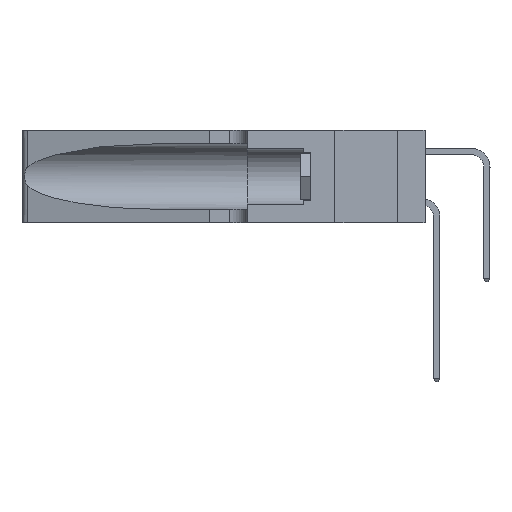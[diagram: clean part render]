
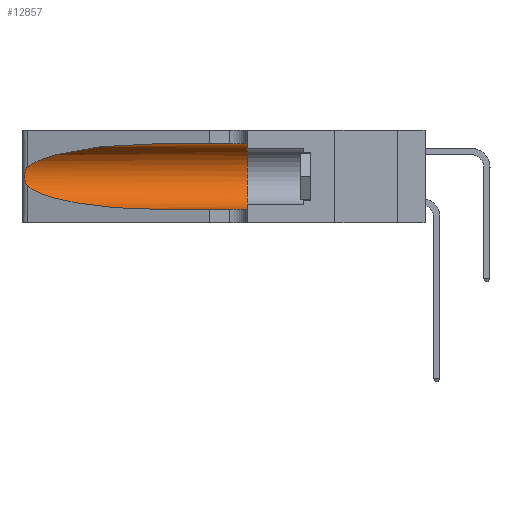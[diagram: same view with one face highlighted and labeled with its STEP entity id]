
A CAD part, left-side view. The second image highlights one B-rep face of the part: STEP entity #12857.
In plain terms, the highlighted cylindrical face has radius 3.308 mm (diameter 6.617 mm), a partial arc.
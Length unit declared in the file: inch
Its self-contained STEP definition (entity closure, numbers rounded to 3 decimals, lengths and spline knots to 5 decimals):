
#152 = CARTESIAN_POINT ( 'NONE',  ( 0.1305, 0.72297, 0.31525 ) ) ;
#205 = DIRECTION ( 'NONE',  ( 0., -1., 0. ) ) ;
#303 =( BOUNDED_CURVE ( )  B_SPLINE_CURVE ( 3, ( #8955, #23123, #22977, #10603 ),
 .UNSPECIFIED., .F., .F. ) 
 B_SPLINE_CURVE_WITH_KNOTS ( ( 4, 4 ),
 ( 3.44316, 4.71239 ),
 .UNSPECIFIED. ) 
 CURVE ( )  GEOMETRIC_REPRESENTATION_ITEM ( )  RATIONAL_B_SPLINE_CURVE ( ( 1., 0.87, 0.87, 1. ) ) 
 REPRESENTATION_ITEM ( '' )  );
#455 = ORIENTED_EDGE ( 'NONE', *, *, #1538, .T. ) ;
#816 = VERTEX_POINT ( 'NONE', #21031 ) ;
#879 = VERTEX_POINT ( 'NONE', #2943 ) ;
#1538 = EDGE_CURVE ( 'NONE', #21488, #879, #303, .T. ) ;
#2738 = CARTESIAN_POINT ( 'NONE',  ( 0.25787, 1.23484, 0.2124 ) ) ;
#2943 = CARTESIAN_POINT ( 'NONE',  ( 0.1305, 0.72297, 0.05475 ) ) ;
#3172 = LINE ( 'NONE', #18869, #17789 ) ;
#3259 = CARTESIAN_POINT ( 'NONE',  ( 0.1305, 0.35, 0.185 ) ) ;
#3769 = ORIENTED_EDGE ( 'NONE', *, *, #12923, .F. ) ;
#3780 = CARTESIAN_POINT ( 'NONE',  ( 0.1305, 1.61858, 0.185 ) ) ;
#3948 = EDGE_CURVE ( 'NONE', #11998, #21488, #16989, .T. ) ;
#4859 = CARTESIAN_POINT ( 'NONE',  ( 0.25487, 1.22718, 0.22369 ) ) ;
#5611 = CARTESIAN_POINT ( 'NONE',  ( 0.2373, 1.15595, 0.28018 ) ) ;
#5813 = CARTESIAN_POINT ( 'NONE',  ( 0.25555, 1.22994, 0.2215 ) ) ;
#6123 = CARTESIAN_POINT ( 'NONE',  ( 0.25487, 1.22718, 0.14631 ) ) ;
#6189 = CARTESIAN_POINT ( 'NONE',  ( 0.26075, 1.23896, 0.19203 ) ) ;
#6513 = VECTOR ( 'NONE', #13451, 39.37008 ) ;
#6566 = DIRECTION ( 'NONE',  ( 0., 0., 1. ) ) ;
#6598 = CARTESIAN_POINT ( 'NONE',  ( 0.25487, 1.22718, 0.14631 ) ) ;
#7074 = AXIS2_PLACEMENT_3D ( 'NONE', #3780, #205, #16344 ) ;
#7425 = ORIENTED_EDGE ( 'NONE', *, *, #15372, .T. ) ;
#8955 = CARTESIAN_POINT ( 'NONE',  ( 0.25487, 1.22718, 0.14631 ) ) ;
#9643 = CARTESIAN_POINT ( 'NONE',  ( 0.25639, 1.23186, 0.15144 ) ) ;
#10056 = EDGE_CURVE ( 'NONE', #22602, #16866, #3172, .T. ) ;
#10603 = CARTESIAN_POINT ( 'NONE',  ( 0.1305, 0.72297, 0.05475 ) ) ;
#10726 = CIRCLE ( 'NONE', #23061, 0.13025 ) ;
#11602 = CARTESIAN_POINT ( 'NONE',  ( 0.25854, 1.2359, 0.20912 ) ) ;
#11998 = VERTEX_POINT ( 'NONE', #4859 ) ;
#12274 = ORIENTED_EDGE ( 'NONE', *, *, #3948, .T. ) ;
#12713 = LINE ( 'NONE', #17176, #6513 ) ;
#12857 = ADVANCED_FACE ( 'NONE', ( #20572 ), #22542, .F. ) ;
#12923 = EDGE_CURVE ( 'NONE', #16866, #816, #10726, .T. ) ;
#13255 = CARTESIAN_POINT ( 'NONE',  ( 0.26075, 1.23896, 0.178 ) ) ;
#13412 = CARTESIAN_POINT ( 'NONE',  ( 0.25789, 1.23486, 0.15765 ) ) ;
#13451 = DIRECTION ( 'NONE',  ( 0., -1., 0. ) ) ;
#14399 = CARTESIAN_POINT ( 'NONE',  ( 0.25487, 1.22718, 0.22369 ) ) ;
#14668 = CARTESIAN_POINT ( 'NONE',  ( 0.25487, 1.22718, 0.22369 ) ) ;
#14923 = DIRECTION ( 'NONE',  ( 0., -1., 0. ) ) ;
#15188 = CARTESIAN_POINT ( 'NONE',  ( 0.25555, 1.22993, 0.14849 ) ) ;
#15372 = EDGE_CURVE ( 'NONE', #22602, #11998, #20162, .T. ) ;
#16290 = CARTESIAN_POINT ( 'NONE',  ( 0.18966, 0.96281, 0.31525 ) ) ;
#16344 = DIRECTION ( 'NONE',  ( 0., 0., -1. ) ) ;
#16866 = VERTEX_POINT ( 'NONE', #20502 ) ;
#16989 = B_SPLINE_CURVE_WITH_KNOTS ( 'NONE', 3,
 ( #14668, #5813, #20590, #2738, #11602, #22480, #6189, #13255, #20437, #18846, #13412, #9643, #15188, #6123 ),
 .UNSPECIFIED., .F., .F.,
 ( 4, 2, 2, 2, 2, 2, 4 ),
 ( 0., 0.00027, 0.00053, 0.00107, 0.0016, 0.00187, 0.00214 ),
 .UNSPECIFIED. ) ;
#17176 = CARTESIAN_POINT ( 'NONE',  ( 0.1305, 1.61858, 0.05475 ) ) ;
#17789 = VECTOR ( 'NONE', #14923, 39.37008 ) ;
#18072 = ORIENTED_EDGE ( 'NONE', *, *, #18517, .T. ) ;
#18517 = EDGE_CURVE ( 'NONE', #879, #816, #12713, .T. ) ;
#18846 = CARTESIAN_POINT ( 'NONE',  ( 0.25856, 1.23593, 0.16098 ) ) ;
#18869 = CARTESIAN_POINT ( 'NONE',  ( 0.1305, 1.61858, 0.31525 ) ) ;
#19788 = CARTESIAN_POINT ( 'NONE',  ( 0.1305, 0.72297, 0.31525 ) ) ;
#20162 =( BOUNDED_CURVE ( )  B_SPLINE_CURVE ( 3, ( #152, #16290, #5611, #14399 ),
 .UNSPECIFIED., .F., .F. ) 
 B_SPLINE_CURVE_WITH_KNOTS ( ( 4, 4 ),
 ( 1.5708, 2.84003 ),
 .UNSPECIFIED. ) 
 CURVE ( )  GEOMETRIC_REPRESENTATION_ITEM ( )  RATIONAL_B_SPLINE_CURVE ( ( 1., 0.87, 0.87, 1. ) ) 
 REPRESENTATION_ITEM ( '' )  );
#20437 = CARTESIAN_POINT ( 'NONE',  ( 0.26017, 1.23833, 0.17102 ) ) ;
#20502 = CARTESIAN_POINT ( 'NONE',  ( 0.1305, 0.35, 0.31525 ) ) ;
#20572 = FACE_OUTER_BOUND ( 'NONE', #22005, .T. ) ;
#20590 = CARTESIAN_POINT ( 'NONE',  ( 0.25639, 1.23184, 0.21858 ) ) ;
#20868 = DIRECTION ( 'NONE',  ( 0., 1., 0. ) ) ;
#21031 = CARTESIAN_POINT ( 'NONE',  ( 0.1305, 0.35, 0.05475 ) ) ;
#21488 = VERTEX_POINT ( 'NONE', #6598 ) ;
#22005 = EDGE_LOOP ( 'NONE', ( #7425, #12274, #455, #18072, #3769, #22765 ) ) ;
#22480 = CARTESIAN_POINT ( 'NONE',  ( 0.26018, 1.23835, 0.19895 ) ) ;
#22542 = CYLINDRICAL_SURFACE ( 'NONE', #7074, 0.13025 ) ;
#22602 = VERTEX_POINT ( 'NONE', #19788 ) ;
#22765 = ORIENTED_EDGE ( 'NONE', *, *, #10056, .F. ) ;
#22977 = CARTESIAN_POINT ( 'NONE',  ( 0.18966, 0.96281, 0.05475 ) ) ;
#23061 = AXIS2_PLACEMENT_3D ( 'NONE', #3259, #20868, #6566 ) ;
#23123 = CARTESIAN_POINT ( 'NONE',  ( 0.2373, 1.15595, 0.08982 ) ) ;
